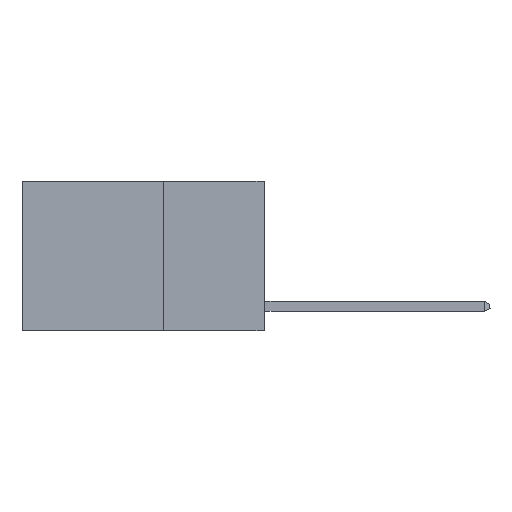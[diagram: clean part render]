
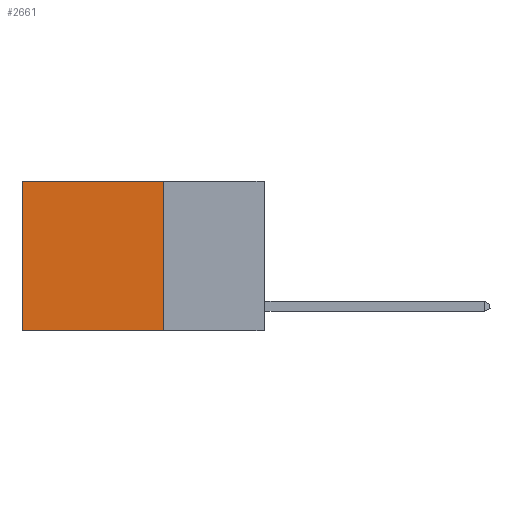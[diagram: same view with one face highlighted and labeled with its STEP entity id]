
A CAD part, left-side view. The second image highlights one B-rep face of the part: STEP entity #2661.
In plain terms, the highlighted planar face has unit normal (-1, 0, 0).
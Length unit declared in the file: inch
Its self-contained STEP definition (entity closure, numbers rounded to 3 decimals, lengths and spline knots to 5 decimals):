
#479 = LINE ( 'NONE', #5381, #14101 ) ;
#480 = CARTESIAN_POINT ( 'NONE',  ( 0.2625, 0.6, 0. ) ) ;
#2037 = VERTEX_POINT ( 'NONE', #4042 ) ;
#2661 = ADVANCED_FACE ( 'NONE', ( #8525 ), #9807, .F. ) ;
#3126 = VERTEX_POINT ( 'NONE', #13463 ) ;
#3492 = CARTESIAN_POINT ( 'NONE',  ( 0.2625, 0.25, 0. ) ) ;
#3757 = DIRECTION ( 'NONE',  ( 1., 0., 0. ) ) ;
#4042 = CARTESIAN_POINT ( 'NONE',  ( 0.2625, 0.6, 0. ) ) ;
#4694 = VECTOR ( 'NONE', #6801, 39.37008 ) ;
#4929 = EDGE_CURVE ( 'NONE', #11652, #2037, #479, .T. ) ;
#4988 = CARTESIAN_POINT ( 'NONE',  ( 0.2625, 0.6, -0.37 ) ) ;
#5381 = CARTESIAN_POINT ( 'NONE',  ( 0.2625, 0.25, 0. ) ) ;
#5384 = VECTOR ( 'NONE', #5964, 39.37008 ) ;
#5926 = CARTESIAN_POINT ( 'NONE',  ( 0.2625, 0.25, 0. ) ) ;
#5964 = DIRECTION ( 'NONE',  ( 0., 0., -1. ) ) ;
#6646 = LINE ( 'NONE', #480, #4694 ) ;
#6801 = DIRECTION ( 'NONE',  ( 0., 0., -1. ) ) ;
#7557 = LINE ( 'NONE', #14676, #12549 ) ;
#8412 = ORIENTED_EDGE ( 'NONE', *, *, #12178, .F. ) ;
#8514 = DIRECTION ( 'NONE',  ( 0., 1., 0. ) ) ;
#8525 = FACE_OUTER_BOUND ( 'NONE', #10740, .T. ) ;
#8601 = DIRECTION ( 'NONE',  ( 0., 0., -1. ) ) ;
#9691 = LINE ( 'NONE', #3492, #5384 ) ;
#9807 = PLANE ( 'NONE',  #14456 ) ;
#10740 = EDGE_LOOP ( 'NONE', ( #14510, #8412, #10999, #13366 ) ) ;
#10999 = ORIENTED_EDGE ( 'NONE', *, *, #11257, .F. ) ;
#11257 = EDGE_CURVE ( 'NONE', #11652, #3126, #9691, .T. ) ;
#11652 = VERTEX_POINT ( 'NONE', #5926 ) ;
#12178 = EDGE_CURVE ( 'NONE', #3126, #15678, #7557, .T. ) ;
#12549 = VECTOR ( 'NONE', #8514, 39.37008 ) ;
#13366 = ORIENTED_EDGE ( 'NONE', *, *, #4929, .T. ) ;
#13463 = CARTESIAN_POINT ( 'NONE',  ( 0.2625, 0.25, -0.37 ) ) ;
#13870 = EDGE_CURVE ( 'NONE', #2037, #15678, #6646, .T. ) ;
#14101 = VECTOR ( 'NONE', #14879, 39.37008 ) ;
#14456 = AXIS2_PLACEMENT_3D ( 'NONE', #14689, #3757, #8601 ) ;
#14510 = ORIENTED_EDGE ( 'NONE', *, *, #13870, .T. ) ;
#14676 = CARTESIAN_POINT ( 'NONE',  ( 0.2625, 0.25, -0.37 ) ) ;
#14689 = CARTESIAN_POINT ( 'NONE',  ( 0.2625, 0.25, 0. ) ) ;
#14879 = DIRECTION ( 'NONE',  ( 0., 1., 0. ) ) ;
#15678 = VERTEX_POINT ( 'NONE', #4988 ) ;
